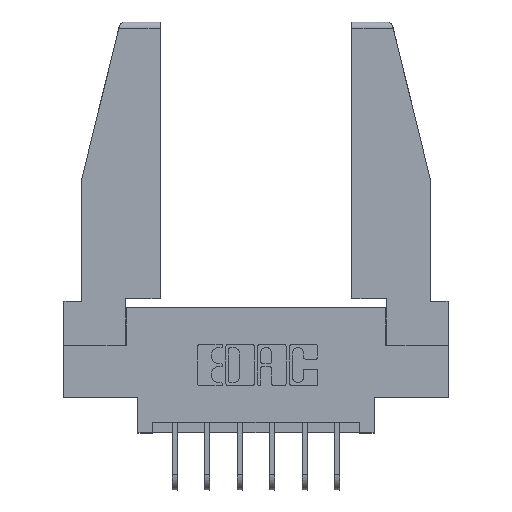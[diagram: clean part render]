
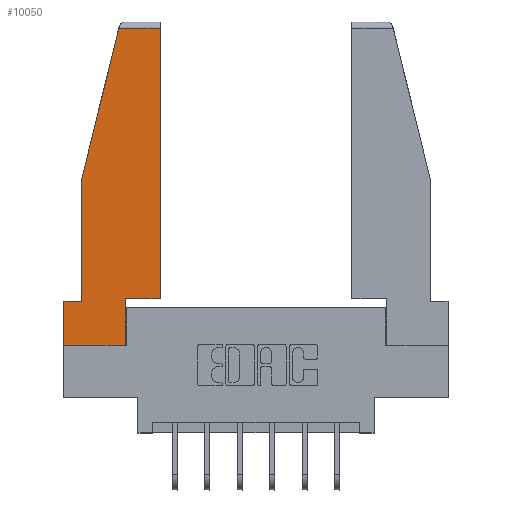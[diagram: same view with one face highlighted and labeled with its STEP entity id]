
A CAD part, top view. The second image highlights one B-rep face of the part: STEP entity #10050.
In plain terms, the highlighted planar face has unit normal (0, 0, 1).
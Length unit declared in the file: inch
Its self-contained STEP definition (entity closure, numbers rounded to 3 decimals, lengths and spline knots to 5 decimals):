
#71 = VERTEX_POINT ( 'NONE', #6768 ) ;
#224 = VECTOR ( 'NONE', #4873, 39.37008 ) ;
#276 = ORIENTED_EDGE ( 'NONE', *, *, #4297, .T. ) ;
#368 = CARTESIAN_POINT ( 'NONE',  ( 0.086, 0.21, 0. ) ) ;
#409 = CARTESIAN_POINT ( 'NONE',  ( 0.297, 0.223, 0. ) ) ;
#435 = DIRECTION ( 'NONE',  ( 0., 1., 0. ) ) ;
#509 = CARTESIAN_POINT ( 'NONE',  ( 0.461, 0.223, 0. ) ) ;
#665 = VECTOR ( 'NONE', #7711, 39.37008 ) ;
#810 = FACE_OUTER_BOUND ( 'NONE', #2775, .T. ) ;
#953 = DIRECTION ( 'NONE',  ( -1., 0., 0. ) ) ;
#1560 = VERTEX_POINT ( 'NONE', #3014 ) ;
#1575 = EDGE_CURVE ( 'NONE', #8324, #7649, #7554, .T. ) ;
#1719 = ORIENTED_EDGE ( 'NONE', *, *, #9200, .T. ) ;
#1808 = VERTEX_POINT ( 'NONE', #4034 ) ;
#2215 = ORIENTED_EDGE ( 'NONE', *, *, #9818, .T. ) ;
#2485 = CARTESIAN_POINT ( 'NONE',  ( 0., 0., 0. ) ) ;
#2539 = ORIENTED_EDGE ( 'NONE', *, *, #9281, .T. ) ;
#2753 = VERTEX_POINT ( 'NONE', #8396 ) ;
#2775 = EDGE_LOOP ( 'NONE', ( #8008, #2215, #6603, #2539, #5928, #11340, #1719, #276, #4014 ) ) ;
#2928 = LINE ( 'NONE', #11642, #11037 ) ;
#2942 = CARTESIAN_POINT ( 'NONE',  ( 0., 0.21, 0. ) ) ;
#3014 = CARTESIAN_POINT ( 'NONE',  ( 0.2636, 1.52, 0. ) ) ;
#3064 = LINE ( 'NONE', #8549, #665 ) ;
#3469 = DIRECTION ( 'NONE',  ( 1., 0., 0. ) ) ;
#3967 = DIRECTION ( 'NONE',  ( 0., -1., 0. ) ) ;
#4014 = ORIENTED_EDGE ( 'NONE', *, *, #4517, .T. ) ;
#4034 = CARTESIAN_POINT ( 'NONE',  ( 0.461, 0.223, 0. ) ) ;
#4053 = EDGE_CURVE ( 'NONE', #4668, #8324, #10232, .T. ) ;
#4297 = EDGE_CURVE ( 'NONE', #7754, #6510, #10919, .T. ) ;
#4517 = EDGE_CURVE ( 'NONE', #6510, #1808, #11484, .T. ) ;
#4666 = LINE ( 'NONE', #509, #9494 ) ;
#4668 = VERTEX_POINT ( 'NONE', #368 ) ;
#4844 = DIRECTION ( 'NONE',  ( 0., 1., 0. ) ) ;
#4873 = DIRECTION ( 'NONE',  ( -0.239, -0.971, 0. ) ) ;
#5380 = VECTOR ( 'NONE', #953, 39.37008 ) ;
#5751 = CARTESIAN_POINT ( 'NONE',  ( 0.297, 0., 0. ) ) ;
#5928 = ORIENTED_EDGE ( 'NONE', *, *, #4053, .T. ) ;
#5930 = VECTOR ( 'NONE', #4844, 39.37008 ) ;
#6241 = DIRECTION ( 'NONE',  ( 0., 0., 1. ) ) ;
#6510 = VERTEX_POINT ( 'NONE', #409 ) ;
#6603 = ORIENTED_EDGE ( 'NONE', *, *, #8558, .T. ) ;
#6768 = CARTESIAN_POINT ( 'NONE',  ( 0.461, 1.52, 0. ) ) ;
#6769 = LINE ( 'NONE', #9512, #7481 ) ;
#6969 = DIRECTION ( 'NONE',  ( 0., -1., 0. ) ) ;
#7176 = CARTESIAN_POINT ( 'NONE',  ( 0.297, 0.223, 0. ) ) ;
#7201 = EDGE_CURVE ( 'NONE', #1808, #71, #4666, .T. ) ;
#7307 = CARTESIAN_POINT ( 'NONE',  ( 0., 0.21, 0. ) ) ;
#7481 = VECTOR ( 'NONE', #11354, 39.37008 ) ;
#7554 = LINE ( 'NONE', #2942, #9836 ) ;
#7649 = VERTEX_POINT ( 'NONE', #2485 ) ;
#7711 = DIRECTION ( 'NONE',  ( -1., 0., 0. ) ) ;
#7754 = VERTEX_POINT ( 'NONE', #8124 ) ;
#8008 = ORIENTED_EDGE ( 'NONE', *, *, #7201, .T. ) ;
#8028 = PLANE ( 'NONE',  #9093 ) ;
#8124 = CARTESIAN_POINT ( 'NONE',  ( 0.297, 0., 0. ) ) ;
#8324 = VERTEX_POINT ( 'NONE', #7307 ) ;
#8396 = CARTESIAN_POINT ( 'NONE',  ( 0.086, 0.8, 0. ) ) ;
#8549 = CARTESIAN_POINT ( 'NONE',  ( 0., 1.52, 0. ) ) ;
#8558 = EDGE_CURVE ( 'NONE', #1560, #2753, #11310, .T. ) ;
#8827 = CARTESIAN_POINT ( 'NONE',  ( 0., 0., 0. ) ) ;
#9093 = AXIS2_PLACEMENT_3D ( 'NONE', #8827, #6241, #3469 ) ;
#9200 = EDGE_CURVE ( 'NONE', #7649, #7754, #6769, .T. ) ;
#9281 = EDGE_CURVE ( 'NONE', #2753, #4668, #2928, .T. ) ;
#9494 = VECTOR ( 'NONE', #435, 39.37008 ) ;
#9512 = CARTESIAN_POINT ( 'NONE',  ( 0., 0., 0. ) ) ;
#9632 = VECTOR ( 'NONE', #10258, 39.37008 ) ;
#9818 = EDGE_CURVE ( 'NONE', #71, #1560, #3064, .T. ) ;
#9836 = VECTOR ( 'NONE', #3967, 39.37008 ) ;
#10050 = ADVANCED_FACE ( 'NONE', ( #810 ), #8028, .T. ) ;
#10232 = LINE ( 'NONE', #10836, #5380 ) ;
#10258 = DIRECTION ( 'NONE',  ( 1., 0., 0. ) ) ;
#10454 = CARTESIAN_POINT ( 'NONE',  ( 0.271, 1.55, 0. ) ) ;
#10836 = CARTESIAN_POINT ( 'NONE',  ( 0., 0.21, 0. ) ) ;
#10919 = LINE ( 'NONE', #5751, #5930 ) ;
#11037 = VECTOR ( 'NONE', #6969, 39.37008 ) ;
#11310 = LINE ( 'NONE', #10454, #224 ) ;
#11340 = ORIENTED_EDGE ( 'NONE', *, *, #1575, .T. ) ;
#11354 = DIRECTION ( 'NONE',  ( 1., 0., 0. ) ) ;
#11484 = LINE ( 'NONE', #7176, #9632 ) ;
#11642 = CARTESIAN_POINT ( 'NONE',  ( 0.086, 0.8, 0. ) ) ;
